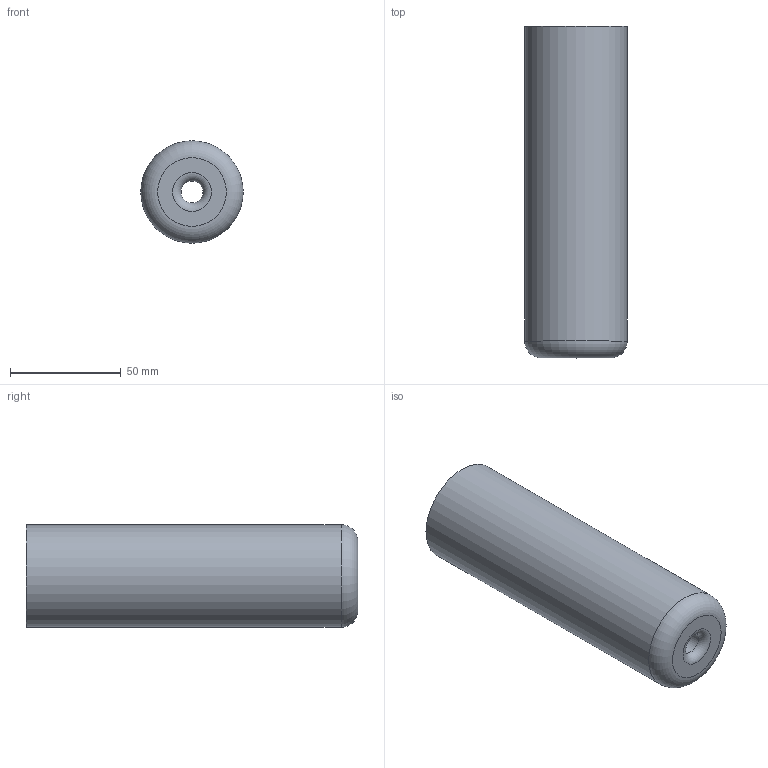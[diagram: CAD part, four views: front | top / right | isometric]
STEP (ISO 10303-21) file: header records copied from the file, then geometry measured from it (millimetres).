
FILE_DESCRIPTION((' '),'2;1');
FILE_NAME('Hydrabarrel3.stp','2013-06-04T21:40:10',(' '),(' '),' ','ACIS',' ');
FILE_SCHEMA(('CONFIG_CONTROL_DESIGN'));
Length unit declared in the file: inch
Products named in the file (1): Hydrabarrel3.stp
Bounding box: 46.28 x 149.86 x 46.28 mm (x, y, z)
Volume: 237956.5 mm3; surface area: 29303.5 mm2
Topology: 1 solids, 1 shells, 14 faces, 22 edges, 14 vertices
Faces by surface type: plane 6, bspline 4, torus 2, cylinder 2
Full cylindrical faces by diameter (mm): 9.906 x1, 46.279 x1
Entity records: 557 total; most frequent: CARTESIAN_POINT 219, DIRECTION 50, ORIENTED_EDGE 28, EDGE_LOOP 28, AXIS2_PLACEMENT_3D 25, VERTEX_POINT 14, CIRCLE 14, EDGE_CURVE 14
